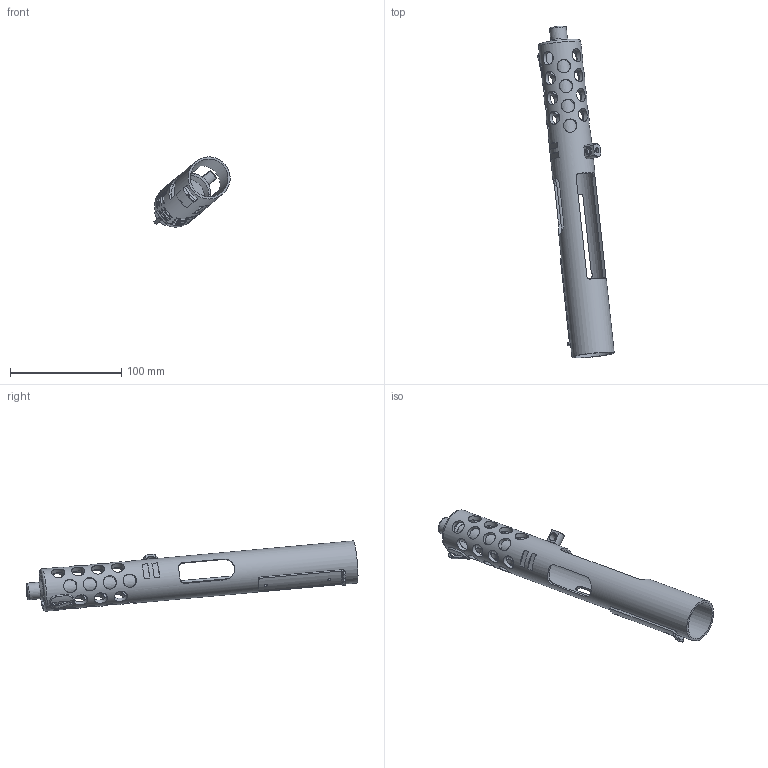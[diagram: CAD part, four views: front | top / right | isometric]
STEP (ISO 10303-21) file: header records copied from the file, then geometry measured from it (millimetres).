
FILE_DESCRIPTION(/* description */ (''),/* implementation_level */ '2;1');
FILE_NAME(/* name */ 'DC9.step',/* time_stamp */ '2025-06-07T20:17:37-04:00',/* author */ (''),/* organization */ (''),/* preprocessor_version */ 'ST-DEVELOPER v20.1',/* originating_system */ 'Autodesk Translation Framework v14.10.0.0',/* authorisation */ '');
FILE_SCHEMA (('AUTOMOTIVE_DESIGN { 1 0 10303 214 3 1 1 }'));
Length unit declared in the file: millimetre
Products named in the file (1): DC9 v1 (1)
Bounding box: 68.66 x 298.27 x 63.18 mm (x, y, z)
Volume: 77136.5 mm3; surface area: 70088.6 mm2
Topology: 7 solids, 7 shells, 153 faces, 450 edges, 311 vertices
Faces by surface type: cylinder 76, plane 55, bspline 14, cone 6, torus 2
Full cylindrical faces by diameter (mm): 5 x2, 7 x1, 8 x1, 9 x3, 12 x31, 15 x2, 16.938 x1, 19.791 x1, 30.1 x1, 34.1 x2, 38.1 x1
Entity records: 10243 total; most frequent: CARTESIAN_POINT 6262, ORIENTED_EDGE 900, DIRECTION 627, EDGE_CURVE 450, VERTEX_POINT 311, EDGE_LOOP 237, AXIS2_PLACEMENT_3D 229, B_SPLINE_CURVE_WITH_KNOTS 188
